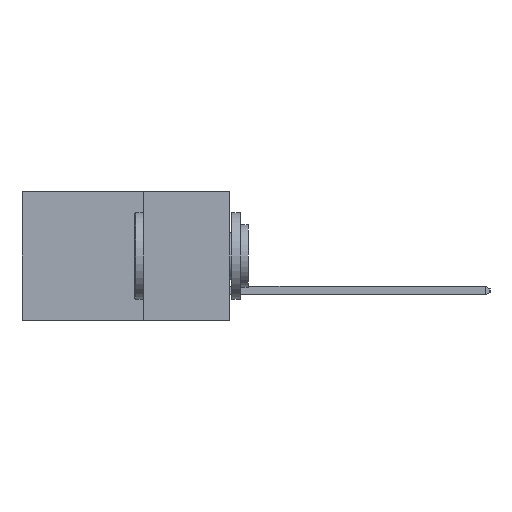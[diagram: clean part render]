
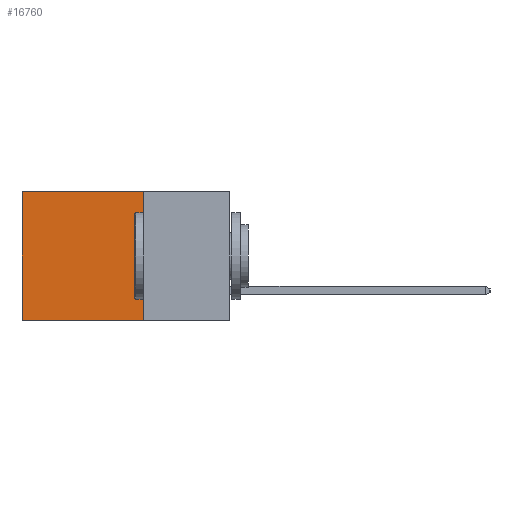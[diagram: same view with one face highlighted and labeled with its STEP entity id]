
A CAD part, left-side view. The second image highlights one B-rep face of the part: STEP entity #16760.
In plain terms, the highlighted planar face has unit normal (-1, 0, 0).
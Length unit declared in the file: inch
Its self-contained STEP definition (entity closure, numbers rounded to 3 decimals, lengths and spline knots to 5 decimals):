
#544 = LINE ( 'NONE', #29421, #25818 ) ;
#1138 = CARTESIAN_POINT ( 'NONE',  ( 0.298, 0.6, 0. ) ) ;
#1496 = EDGE_CURVE ( 'NONE', #29123, #2514, #544, .T. ) ;
#2514 = VERTEX_POINT ( 'NONE', #20541 ) ;
#2624 = LINE ( 'NONE', #1138, #22052 ) ;
#5697 = PLANE ( 'NONE',  #21387 ) ;
#6165 = DIRECTION ( 'NONE',  ( 0., 0., -1. ) ) ;
#8114 = ORIENTED_EDGE ( 'NONE', *, *, #15954, .F. ) ;
#8131 = DIRECTION ( 'NONE',  ( 1., 0., 0. ) ) ;
#8712 = FACE_OUTER_BOUND ( 'NONE', #9544, .T. ) ;
#9021 = LINE ( 'NONE', #23098, #26934 ) ;
#9535 = LINE ( 'NONE', #24125, #22450 ) ;
#9544 = EDGE_LOOP ( 'NONE', ( #25907, #8114, #21793, #10405 ) ) ;
#10405 = ORIENTED_EDGE ( 'NONE', *, *, #18366, .T. ) ;
#11604 = EDGE_CURVE ( 'NONE', #12875, #28047, #2624, .T. ) ;
#12875 = VERTEX_POINT ( 'NONE', #15632 ) ;
#12995 = CARTESIAN_POINT ( 'NONE',  ( 0.298, 0.6, -0.37 ) ) ;
#13436 = DIRECTION ( 'NONE',  ( 0., 1., 0. ) ) ;
#14852 = CARTESIAN_POINT ( 'NONE',  ( 0.298, 0.25, 0. ) ) ;
#15632 = CARTESIAN_POINT ( 'NONE',  ( 0.298, 0.6, 0. ) ) ;
#15954 = EDGE_CURVE ( 'NONE', #2514, #28047, #9535, .T. ) ;
#16756 = DIRECTION ( 'NONE',  ( 0., 1., 0. ) ) ;
#16760 = ADVANCED_FACE ( 'NONE', ( #8712 ), #5697, .F. ) ;
#17960 = DIRECTION ( 'NONE',  ( 0., 0., -1. ) ) ;
#18366 = EDGE_CURVE ( 'NONE', #29123, #12875, #9021, .T. ) ;
#20541 = CARTESIAN_POINT ( 'NONE',  ( 0.298, 0.25, -0.37 ) ) ;
#21387 = AXIS2_PLACEMENT_3D ( 'NONE', #22678, #8131, #25156 ) ;
#21793 = ORIENTED_EDGE ( 'NONE', *, *, #1496, .F. ) ;
#22052 = VECTOR ( 'NONE', #6165, 39.37008 ) ;
#22450 = VECTOR ( 'NONE', #16756, 39.37008 ) ;
#22678 = CARTESIAN_POINT ( 'NONE',  ( 0.298, 0.25, 0. ) ) ;
#23098 = CARTESIAN_POINT ( 'NONE',  ( 0.298, 0.25, 0. ) ) ;
#24125 = CARTESIAN_POINT ( 'NONE',  ( 0.298, 0.25, -0.37 ) ) ;
#25156 = DIRECTION ( 'NONE',  ( 0., 0., -1. ) ) ;
#25818 = VECTOR ( 'NONE', #17960, 39.37008 ) ;
#25907 = ORIENTED_EDGE ( 'NONE', *, *, #11604, .T. ) ;
#26934 = VECTOR ( 'NONE', #13436, 39.37008 ) ;
#28047 = VERTEX_POINT ( 'NONE', #12995 ) ;
#29123 = VERTEX_POINT ( 'NONE', #14852 ) ;
#29421 = CARTESIAN_POINT ( 'NONE',  ( 0.298, 0.25, 0. ) ) ;
